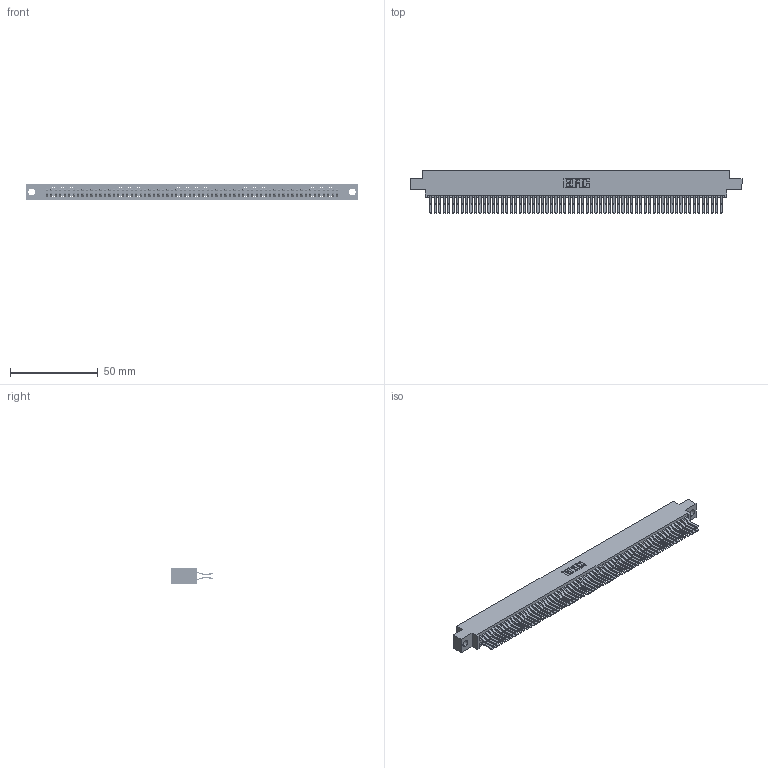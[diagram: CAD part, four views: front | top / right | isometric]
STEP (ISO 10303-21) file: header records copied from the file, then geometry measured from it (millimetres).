
FILE_DESCRIPTION (( 'STEP AP203' ), '1' );
FILE_NAME ('395-132-560-804.STEP', '2021-06-18T01:34:58', ( '' ), ( '' ), 'SwSTEP 2.0', 'SolidWorks 2020', '' );
FILE_SCHEMA (( 'CONFIG_CONTROL_DESIGN' ));
Length unit declared in the file: inch
Products named in the file (3): 395-132-560-804; 345-292-001_560 Tail; 345 Part_0.170 Offset - 0.156 Dia-TI
Assembly tree (133 placements, depth 2):
  395-132-560-804
    345 Part_0.170 Offset - 0.156 Dia-TI
    345-292-001_560 Tail  x132
Bounding box: 188.85 x 24.45 x 9.4 mm (x, y, z)
Volume: 19213.6 mm3; surface area: 31086.1 mm2
Topology: 133 solids, 133 shells, 7008 faces, 20849 edges, 13722 vertices
Faces by surface type: plane 4454, cylinder 2554
Entity records: 49193 total; most frequent: CARTESIAN_POINT 8230, ORIENTED_EDGE 8162, DIRECTION 7229, EDGE_CURVE 4081, VECTOR 3681, LINE 3681, VERTEX_POINT 2718, AXIS2_PLACEMENT_3D 1774
